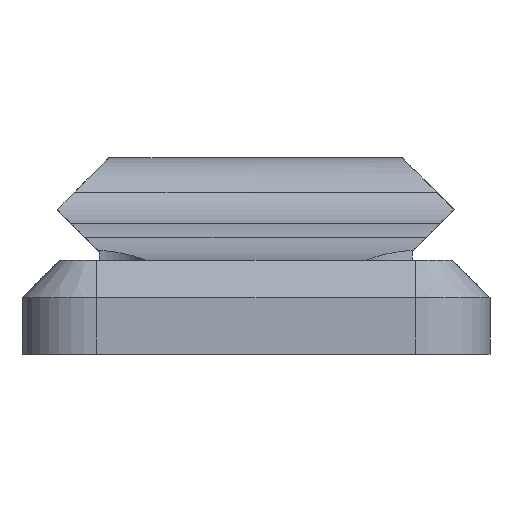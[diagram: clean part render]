
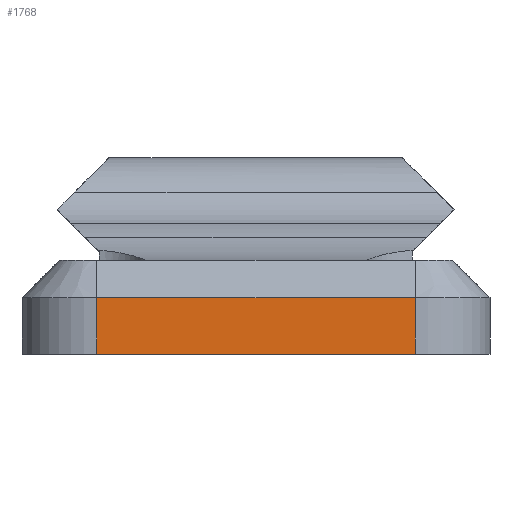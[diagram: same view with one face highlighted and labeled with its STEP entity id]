
A CAD part, front view. The second image highlights one B-rep face of the part: STEP entity #1768.
In plain terms, the highlighted planar face has unit normal (0, -1, 0).
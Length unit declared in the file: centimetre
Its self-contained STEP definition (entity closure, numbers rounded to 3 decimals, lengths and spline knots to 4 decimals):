
#140=PLANE($,#1931);
#215=FACE_OUTER_BOUND($,#317,.T.);
#317=EDGE_LOOP($,(#1596,#1597,#1598,#1599));
#476=LINE($,#2899,#651);
#493=LINE($,#2966,#668);
#502=LINE($,#3003,#677);
#503=LINE($,#3005,#678);
#651=VECTOR($,#2285,1.7);
#668=VECTOR($,#2356,1.7);
#677=VECTOR($,#2397,0.3);
#678=VECTOR($,#2400,0.3);
#855=VERTEX_POINT($,#2893);
#856=VERTEX_POINT($,#2897);
#878=VERTEX_POINT($,#2963);
#879=VERTEX_POINT($,#2965);
#1085=EDGE_CURVE($,#855,#856,#476,.T.);
#1120=EDGE_CURVE($,#878,#879,#493,.T.);
#1138=EDGE_CURVE($,#879,#855,#502,.T.);
#1139=EDGE_CURVE($,#878,#856,#503,.T.);
#1596=ORIENTED_EDGE($,*,*,#1085,.F.);
#1597=ORIENTED_EDGE($,*,*,#1138,.F.);
#1598=ORIENTED_EDGE($,*,*,#1120,.F.);
#1599=ORIENTED_EDGE($,*,*,#1139,.T.);
#1768=ADVANCED_FACE($,(#215),#140,.T.);
#1931=AXIS2_PLACEMENT_3D($,#3004,#2398,#2399);
#2285=DIRECTION($,(1.,0.,0.));
#2356=DIRECTION($,(-1.,0.,0.));
#2397=DIRECTION($,(0.,0.,1.));
#2398=DIRECTION('center_axis',(0.,-1.,0.));
#2399=DIRECTION('ref_axis',(1.,0.,0.));
#2400=DIRECTION($,(0.,0.,1.));
#2893=CARTESIAN_POINT('',(-14.2975,3.0286,12.1775));
#2897=CARTESIAN_POINT('',(-12.5975,3.0286,12.1775));
#2899=CARTESIAN_POINT($,(-13.2385,3.0286,12.1775));
#2963=CARTESIAN_POINT('',(-12.5975,3.0286,11.8775));
#2965=CARTESIAN_POINT('',(-14.2975,3.0286,11.8775));
#2966=CARTESIAN_POINT($,(-14.2538,3.0286,11.8775));
#3003=CARTESIAN_POINT($,(-14.2975,3.0286,12.2775));
#3004=CARTESIAN_POINT('Origin',(-14.2975,3.0286,12.2775));
#3005=CARTESIAN_POINT($,(-12.5975,3.0286,12.2775));
